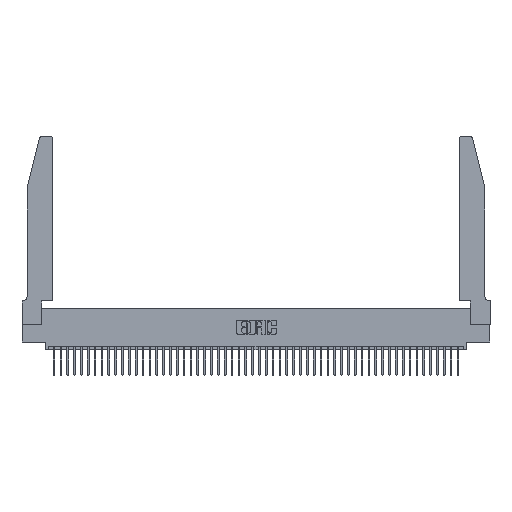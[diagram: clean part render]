
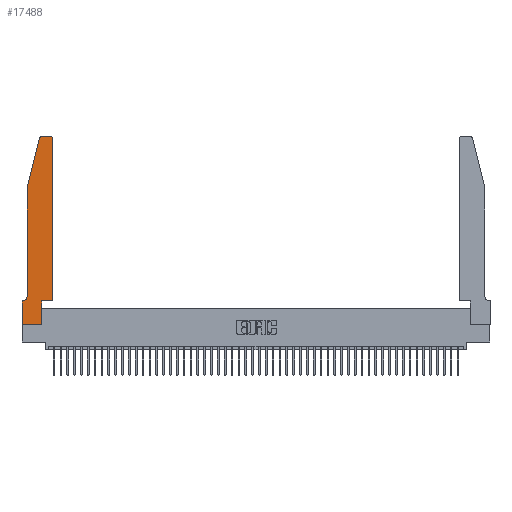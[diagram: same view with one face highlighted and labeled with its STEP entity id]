
A CAD part, top view. The second image highlights one B-rep face of the part: STEP entity #17488.
In plain terms, the highlighted planar face has unit normal (0, 0, 1).
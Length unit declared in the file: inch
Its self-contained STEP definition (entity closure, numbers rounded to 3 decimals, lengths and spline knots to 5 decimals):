
#859 = ORIENTED_EDGE ( 'NONE', *, *, #21460, .T. ) ;
#1425 = LINE ( 'NONE', #16813, #23654 ) ;
#1528 = ORIENTED_EDGE ( 'NONE', *, *, #21483, .T. ) ;
#1682 = AXIS2_PLACEMENT_3D ( 'NONE', #32780, #13687, #21253 ) ;
#2059 = AXIS2_PLACEMENT_3D ( 'NONE', #44197, #43858, #24767 ) ;
#2571 = DIRECTION ( 'NONE',  ( 1., 0., 0. ) ) ;
#2691 = EDGE_CURVE ( 'NONE', #6597, #40697, #21099, .T. ) ;
#3837 = CARTESIAN_POINT ( 'NONE',  ( 0.0755, 2., 0.37 ) ) ;
#4089 = CARTESIAN_POINT ( 'NONE',  ( 0.284, 2.75, 0.37 ) ) ;
#4143 = LINE ( 'NONE', #3837, #18501 ) ;
#4511 = ORIENTED_EDGE ( 'NONE', *, *, #15130, .T. ) ;
#4549 = CIRCLE ( 'NONE', #1682, 0.07 ) ;
#4658 = VERTEX_POINT ( 'NONE', #47118 ) ;
#4781 = FACE_OUTER_BOUND ( 'NONE', #11142, .T. ) ;
#5348 = CARTESIAN_POINT ( 'NONE',  ( 0.4505, 0.35, 0.37 ) ) ;
#5810 = VERTEX_POINT ( 'NONE', #19909 ) ;
#6597 = VERTEX_POINT ( 'NONE', #40450 ) ;
#7697 = VERTEX_POINT ( 'NONE', #31782 ) ;
#7728 = EDGE_CURVE ( 'NONE', #5810, #22123, #4549, .T. ) ;
#7995 = VECTOR ( 'NONE', #2571, 39.37008 ) ;
#8095 = LINE ( 'NONE', #49196, #47627 ) ;
#8344 = DIRECTION ( 'NONE',  ( -1., 0., 0. ) ) ;
#8585 = LINE ( 'NONE', #10582, #7995 ) ;
#8899 = ORIENTED_EDGE ( 'NONE', *, *, #17599, .T. ) ;
#9211 = CARTESIAN_POINT ( 'NONE',  ( 0.4205, 2.75, 0.37 ) ) ;
#10582 = CARTESIAN_POINT ( 'NONE',  ( 0., 0., 0.37 ) ) ;
#11142 = EDGE_LOOP ( 'NONE', ( #1528, #4511, #49104, #21447, #37479, #29348, #859, #36501, #12267, #8899, #40415, #39311 ) ) ;
#11791 = EDGE_CURVE ( 'NONE', #13335, #4658, #4143, .T. ) ;
#12267 = ORIENTED_EDGE ( 'NONE', *, *, #48325, .T. ) ;
#13335 = VERTEX_POINT ( 'NONE', #25154 ) ;
#13687 = DIRECTION ( 'NONE',  ( 0., 0., -1. ) ) ;
#14238 = DIRECTION ( 'NONE',  ( 0., 0., 1. ) ) ;
#14675 = LINE ( 'NONE', #33464, #23689 ) ;
#15130 = EDGE_CURVE ( 'NONE', #34586, #13335, #15826, .T. ) ;
#15384 = LINE ( 'NONE', #15728, #24370 ) ;
#15728 = CARTESIAN_POINT ( 'NONE',  ( 0.0755, 0.35, 0.37 ) ) ;
#15826 = CIRCLE ( 'NONE', #39535, 0.03 ) ;
#16813 = CARTESIAN_POINT ( 'NONE',  ( 0.2865, 0.35, 0.37 ) ) ;
#17169 = CARTESIAN_POINT ( 'NONE',  ( 0.4205, 2.72, 0.37 ) ) ;
#17488 = ADVANCED_FACE ( 'NONE', ( #4781 ), #32774, .T. ) ;
#17599 = EDGE_CURVE ( 'NONE', #40368, #7697, #27502, .T. ) ;
#18501 = VECTOR ( 'NONE', #19071, 39.37008 ) ;
#19071 = DIRECTION ( 'NONE',  ( -0.239, -0.971, 0. ) ) ;
#19909 = CARTESIAN_POINT ( 'NONE',  ( 0.0755, 0.42, 0.37 ) ) ;
#21099 = CIRCLE ( 'NONE', #32985, 0.03 ) ;
#21253 = DIRECTION ( 'NONE',  ( -1., 0., 0. ) ) ;
#21334 = DIRECTION ( 'NONE',  ( 0., 0., 1. ) ) ;
#21447 = ORIENTED_EDGE ( 'NONE', *, *, #41989, .T. ) ;
#21460 = EDGE_CURVE ( 'NONE', #25028, #29660, #32066, .T. ) ;
#21483 = EDGE_CURVE ( 'NONE', #40697, #34586, #8095, .T. ) ;
#21511 = EDGE_CURVE ( 'NONE', #7697, #6597, #14675, .T. ) ;
#22094 = DIRECTION ( 'NONE',  ( -1., 0., 0. ) ) ;
#22123 = VERTEX_POINT ( 'NONE', #45158 ) ;
#23654 = VECTOR ( 'NONE', #28542, 39.37008 ) ;
#23689 = VECTOR ( 'NONE', #45382, 39.37008 ) ;
#24370 = VECTOR ( 'NONE', #8344, 39.37008 ) ;
#24767 = DIRECTION ( 'NONE',  ( 1., 0., 0. ) ) ;
#25028 = VERTEX_POINT ( 'NONE', #49409 ) ;
#25154 = CARTESIAN_POINT ( 'NONE',  ( 0.25487, 2.72718, 0.37 ) ) ;
#25208 = CARTESIAN_POINT ( 'NONE',  ( 0.0755, 2., 0.37 ) ) ;
#25222 = CARTESIAN_POINT ( 'NONE',  ( 0., 0., 0.37 ) ) ;
#27502 = LINE ( 'NONE', #5348, #44275 ) ;
#28542 = DIRECTION ( 'NONE',  ( 0., 1., 0. ) ) ;
#29121 = CARTESIAN_POINT ( 'NONE',  ( 0., 0., 0.37 ) ) ;
#29348 = ORIENTED_EDGE ( 'NONE', *, *, #32751, .T. ) ;
#29660 = VERTEX_POINT ( 'NONE', #25222 ) ;
#29666 = VECTOR ( 'NONE', #41526, 39.37008 ) ;
#31593 = LINE ( 'NONE', #25208, #32209 ) ;
#31782 = CARTESIAN_POINT ( 'NONE',  ( 0.4505, 0.35, 0.37 ) ) ;
#31878 = CARTESIAN_POINT ( 'NONE',  ( 0.2865, 0., 0.37 ) ) ;
#32066 = LINE ( 'NONE', #29121, #29666 ) ;
#32209 = VECTOR ( 'NONE', #32378, 39.37008 ) ;
#32378 = DIRECTION ( 'NONE',  ( 0., -1., 0. ) ) ;
#32751 = EDGE_CURVE ( 'NONE', #22123, #25028, #15384, .T. ) ;
#32774 = PLANE ( 'NONE',  #2059 ) ;
#32780 = CARTESIAN_POINT ( 'NONE',  ( 0.0055, 0.42, 0.37 ) ) ;
#32985 = AXIS2_PLACEMENT_3D ( 'NONE', #17169, #21334, #43960 ) ;
#33273 = DIRECTION ( 'NONE',  ( 1., 0., 0. ) ) ;
#33464 = CARTESIAN_POINT ( 'NONE',  ( 0.4505, 0.35, 0.37 ) ) ;
#33497 = CARTESIAN_POINT ( 'NONE',  ( 0.284, 2.72, 0.37 ) ) ;
#34586 = VERTEX_POINT ( 'NONE', #4089 ) ;
#36501 = ORIENTED_EDGE ( 'NONE', *, *, #48508, .T. ) ;
#37479 = ORIENTED_EDGE ( 'NONE', *, *, #7728, .T. ) ;
#37735 = CARTESIAN_POINT ( 'NONE',  ( 0.2865, 0.35, 0.37 ) ) ;
#39311 = ORIENTED_EDGE ( 'NONE', *, *, #2691, .T. ) ;
#39535 = AXIS2_PLACEMENT_3D ( 'NONE', #33497, #14238, #41240 ) ;
#40368 = VERTEX_POINT ( 'NONE', #37735 ) ;
#40415 = ORIENTED_EDGE ( 'NONE', *, *, #21511, .T. ) ;
#40450 = CARTESIAN_POINT ( 'NONE',  ( 0.4505, 2.72, 0.37 ) ) ;
#40697 = VERTEX_POINT ( 'NONE', #9211 ) ;
#41240 = DIRECTION ( 'NONE',  ( 1., 0., 0. ) ) ;
#41526 = DIRECTION ( 'NONE',  ( 0., -1., 0. ) ) ;
#41989 = EDGE_CURVE ( 'NONE', #4658, #5810, #31593, .T. ) ;
#43663 = VERTEX_POINT ( 'NONE', #31878 ) ;
#43858 = DIRECTION ( 'NONE',  ( 0., 0., 1. ) ) ;
#43960 = DIRECTION ( 'NONE',  ( 1., 0., 0. ) ) ;
#44197 = CARTESIAN_POINT ( 'NONE',  ( 0., 0.35, 0.37 ) ) ;
#44275 = VECTOR ( 'NONE', #33273, 39.37008 ) ;
#45158 = CARTESIAN_POINT ( 'NONE',  ( 0.0055, 0.35, 0.37 ) ) ;
#45382 = DIRECTION ( 'NONE',  ( 0., 1., 0. ) ) ;
#47118 = CARTESIAN_POINT ( 'NONE',  ( 0.0755, 2., 0.37 ) ) ;
#47627 = VECTOR ( 'NONE', #22094, 39.37008 ) ;
#48325 = EDGE_CURVE ( 'NONE', #43663, #40368, #1425, .T. ) ;
#48508 = EDGE_CURVE ( 'NONE', #29660, #43663, #8585, .T. ) ;
#49104 = ORIENTED_EDGE ( 'NONE', *, *, #11791, .T. ) ;
#49196 = CARTESIAN_POINT ( 'NONE',  ( 0.2605, 2.75, 0.37 ) ) ;
#49409 = CARTESIAN_POINT ( 'NONE',  ( 0., 0.35, 0.37 ) ) ;
